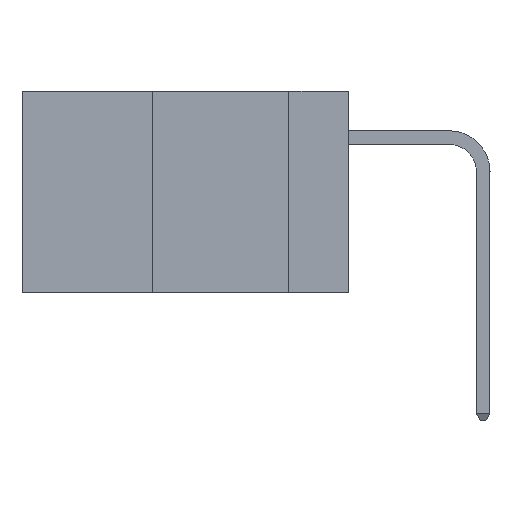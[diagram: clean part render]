
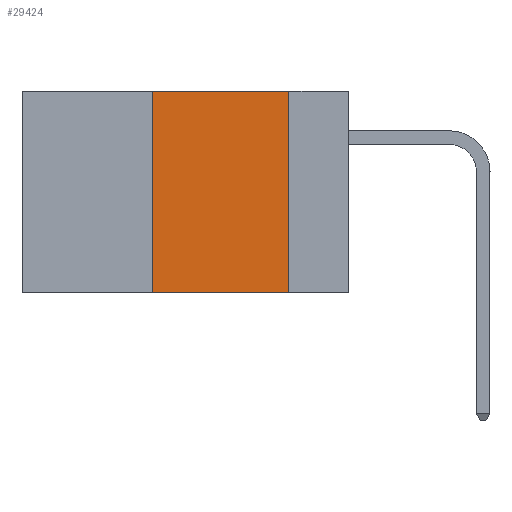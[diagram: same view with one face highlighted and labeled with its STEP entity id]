
A CAD part, left-side view. The second image highlights one B-rep face of the part: STEP entity #29424.
In plain terms, the highlighted planar face has unit normal (-1, 0, 0).
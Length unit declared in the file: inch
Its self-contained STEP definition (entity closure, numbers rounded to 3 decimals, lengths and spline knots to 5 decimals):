
#1412 = DIRECTION ( 'NONE',  ( 0., -1., 0. ) ) ;
#2646 = CARTESIAN_POINT ( 'NONE',  ( 0., 0.11, -0.37 ) ) ;
#3709 = VECTOR ( 'NONE', #1412, 39.37008 ) ;
#3829 = CARTESIAN_POINT ( 'NONE',  ( 0., 0.11, 0. ) ) ;
#4793 = ORIENTED_EDGE ( 'NONE', *, *, #28523, .F. ) ;
#5952 = DIRECTION ( 'NONE',  ( 0., 0., -1. ) ) ;
#6775 = DIRECTION ( 'NONE',  ( 0., 0., -1. ) ) ;
#7477 = EDGE_CURVE ( 'NONE', #26232, #15872, #12270, .T. ) ;
#8387 = DIRECTION ( 'NONE',  ( 0., 0., 1. ) ) ;
#9050 = CARTESIAN_POINT ( 'NONE',  ( 0., 0.6, -0.37 ) ) ;
#10216 = CARTESIAN_POINT ( 'NONE',  ( 0., 0.36, -0.37 ) ) ;
#10349 = CARTESIAN_POINT ( 'NONE',  ( 0., 0.6, 0. ) ) ;
#10729 = LINE ( 'NONE', #9050, #34355 ) ;
#11263 = VECTOR ( 'NONE', #6775, 39.37008 ) ;
#12206 = AXIS2_PLACEMENT_3D ( 'NONE', #17686, #23674, #5952 ) ;
#12270 = LINE ( 'NONE', #26106, #34909 ) ;
#12480 = LINE ( 'NONE', #10349, #3709 ) ;
#15872 = VERTEX_POINT ( 'NONE', #18671 ) ;
#16532 = FACE_OUTER_BOUND ( 'NONE', #37153, .T. ) ;
#17686 = CARTESIAN_POINT ( 'NONE',  ( 0., 0.6, 0. ) ) ;
#18587 = CARTESIAN_POINT ( 'NONE',  ( 0., 0.11, 0. ) ) ;
#18671 = CARTESIAN_POINT ( 'NONE',  ( 0., 0.36, 0. ) ) ;
#19151 = LINE ( 'NONE', #3829, #11263 ) ;
#23534 = EDGE_CURVE ( 'NONE', #29591, #28129, #19151, .T. ) ;
#23674 = DIRECTION ( 'NONE',  ( 1., 0., 0. ) ) ;
#25190 = ORIENTED_EDGE ( 'NONE', *, *, #7477, .F. ) ;
#26106 = CARTESIAN_POINT ( 'NONE',  ( 0., 0.36, 0. ) ) ;
#26232 = VERTEX_POINT ( 'NONE', #10216 ) ;
#27621 = ORIENTED_EDGE ( 'NONE', *, *, #37491, .T. ) ;
#28129 = VERTEX_POINT ( 'NONE', #2646 ) ;
#28523 = EDGE_CURVE ( 'NONE', #15872, #29591, #12480, .T. ) ;
#29424 = ADVANCED_FACE ( 'NONE', ( #16532 ), #32455, .F. ) ;
#29591 = VERTEX_POINT ( 'NONE', #18587 ) ;
#30709 = ORIENTED_EDGE ( 'NONE', *, *, #23534, .F. ) ;
#32455 = PLANE ( 'NONE',  #12206 ) ;
#34355 = VECTOR ( 'NONE', #35701, 39.37008 ) ;
#34909 = VECTOR ( 'NONE', #8387, 39.37008 ) ;
#35701 = DIRECTION ( 'NONE',  ( 0., -1., 0. ) ) ;
#37153 = EDGE_LOOP ( 'NONE', ( #30709, #4793, #25190, #27621 ) ) ;
#37491 = EDGE_CURVE ( 'NONE', #26232, #28129, #10729, .T. ) ;
